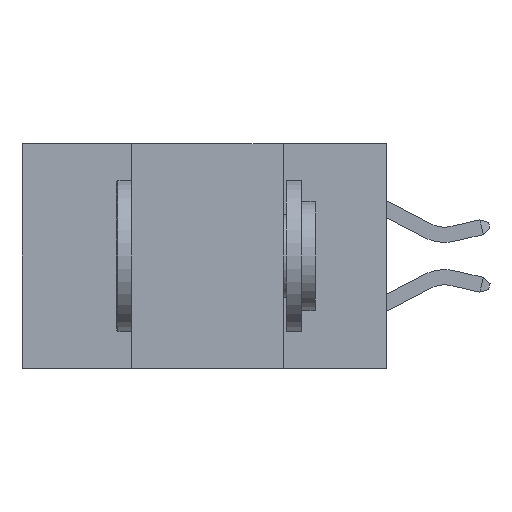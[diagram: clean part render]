
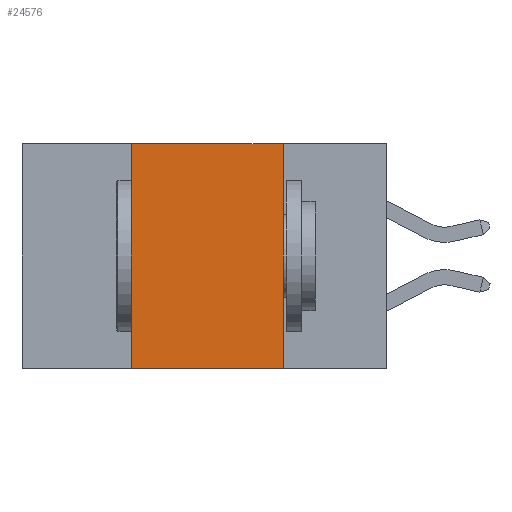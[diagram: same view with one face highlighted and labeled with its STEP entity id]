
A CAD part, left-side view. The second image highlights one B-rep face of the part: STEP entity #24576.
In plain terms, the highlighted planar face has unit normal (-1, 0, 0).
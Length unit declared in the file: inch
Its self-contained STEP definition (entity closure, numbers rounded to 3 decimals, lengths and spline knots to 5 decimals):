
#2789 = VERTEX_POINT ( 'NONE', #16860 ) ;
#4865 = CARTESIAN_POINT ( 'NONE',  ( 0., 0.42, -0.37 ) ) ;
#7009 = VECTOR ( 'NONE', #24957, 39.37008 ) ;
#7039 = LINE ( 'NONE', #17859, #7009 ) ;
#7182 = DIRECTION ( 'NONE',  ( 0., -1., 0. ) ) ;
#7869 = LINE ( 'NONE', #8786, #8589 ) ;
#8450 = VERTEX_POINT ( 'NONE', #28013 ) ;
#8589 = VECTOR ( 'NONE', #20316, 39.37008 ) ;
#8786 = CARTESIAN_POINT ( 'NONE',  ( 0., 0.17, 0. ) ) ;
#9841 = CARTESIAN_POINT ( 'NONE',  ( 0., 0.6, 0. ) ) ;
#9977 = VECTOR ( 'NONE', #7182, 39.37008 ) ;
#10468 = FACE_OUTER_BOUND ( 'NONE', #28235, .T. ) ;
#11290 = DIRECTION ( 'NONE',  ( 0., 0., 1. ) ) ;
#11955 = EDGE_CURVE ( 'NONE', #2789, #30223, #16586, .T. ) ;
#12377 = ORIENTED_EDGE ( 'NONE', *, *, #30068, .F. ) ;
#12404 = AXIS2_PLACEMENT_3D ( 'NONE', #23847, #26500, #28622 ) ;
#12413 = EDGE_CURVE ( 'NONE', #26180, #2789, #21353, .T. ) ;
#16586 = LINE ( 'NONE', #9841, #9977 ) ;
#16860 = CARTESIAN_POINT ( 'NONE',  ( 0., 0.42, 0. ) ) ;
#17859 = CARTESIAN_POINT ( 'NONE',  ( 0., 0.6, -0.37 ) ) ;
#19293 = PLANE ( 'NONE',  #12404 ) ;
#20158 = ORIENTED_EDGE ( 'NONE', *, *, #11955, .F. ) ;
#20316 = DIRECTION ( 'NONE',  ( 0., 0., -1. ) ) ;
#20452 = ORIENTED_EDGE ( 'NONE', *, *, #12413, .F. ) ;
#21353 = LINE ( 'NONE', #29849, #27944 ) ;
#23520 = CARTESIAN_POINT ( 'NONE',  ( 0., 0.17, 0. ) ) ;
#23847 = CARTESIAN_POINT ( 'NONE',  ( 0., 0.6, 0. ) ) ;
#24576 = ADVANCED_FACE ( 'NONE', ( #10468 ), #19293, .F. ) ;
#24902 = ORIENTED_EDGE ( 'NONE', *, *, #26480, .T. ) ;
#24957 = DIRECTION ( 'NONE',  ( 0., -1., 0. ) ) ;
#26180 = VERTEX_POINT ( 'NONE', #4865 ) ;
#26480 = EDGE_CURVE ( 'NONE', #26180, #8450, #7039, .T. ) ;
#26500 = DIRECTION ( 'NONE',  ( 1., 0., 0. ) ) ;
#27944 = VECTOR ( 'NONE', #11290, 39.37008 ) ;
#28013 = CARTESIAN_POINT ( 'NONE',  ( 0., 0.17, -0.37 ) ) ;
#28235 = EDGE_LOOP ( 'NONE', ( #12377, #20158, #20452, #24902 ) ) ;
#28622 = DIRECTION ( 'NONE',  ( 0., 0., -1. ) ) ;
#29849 = CARTESIAN_POINT ( 'NONE',  ( 0., 0.42, 0. ) ) ;
#30068 = EDGE_CURVE ( 'NONE', #30223, #8450, #7869, .T. ) ;
#30223 = VERTEX_POINT ( 'NONE', #23520 ) ;
